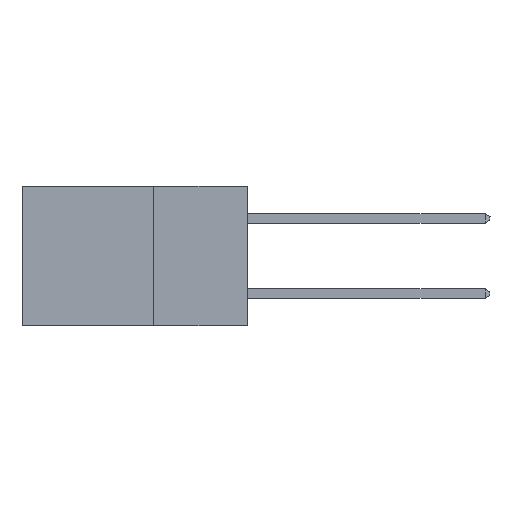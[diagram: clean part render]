
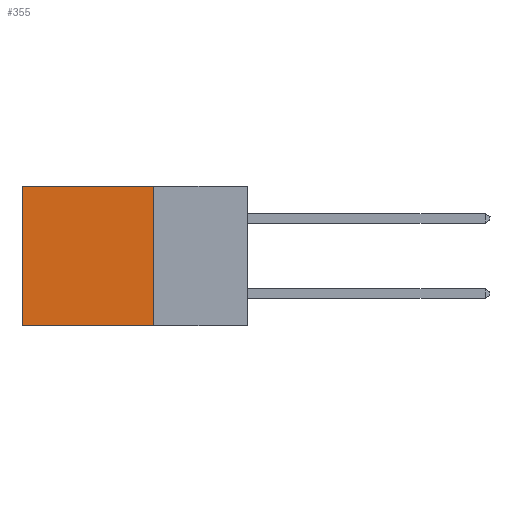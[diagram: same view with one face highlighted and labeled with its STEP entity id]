
A CAD part, left-side view. The second image highlights one B-rep face of the part: STEP entity #355.
In plain terms, the highlighted planar face has unit normal (-1, 0, 0).
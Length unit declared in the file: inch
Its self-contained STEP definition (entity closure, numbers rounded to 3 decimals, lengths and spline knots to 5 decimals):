
#151 = EDGE_CURVE ( 'NONE', #7966, #12110, #7622, .T. ) ;
#355 = ADVANCED_FACE ( 'NONE', ( #9248 ), #10595, .F. ) ;
#1517 = DIRECTION ( 'NONE',  ( 0., 1., 0. ) ) ;
#2015 = EDGE_LOOP ( 'NONE', ( #2437, #8080, #8118, #6639 ) ) ;
#2432 = VERTEX_POINT ( 'NONE', #17488 ) ;
#2437 = ORIENTED_EDGE ( 'NONE', *, *, #8890, .T. ) ;
#2986 = CARTESIAN_POINT ( 'NONE',  ( 0.2615, 0.25, -0.37 ) ) ;
#3216 = VECTOR ( 'NONE', #7838, 39.37008 ) ;
#3565 = DIRECTION ( 'NONE',  ( 1., 0., 0. ) ) ;
#3837 = CARTESIAN_POINT ( 'NONE',  ( 0.2615, 0.25, -0.37 ) ) ;
#6639 = ORIENTED_EDGE ( 'NONE', *, *, #10922, .T. ) ;
#6640 = EDGE_CURVE ( 'NONE', #12110, #2432, #9597, .T. ) ;
#7526 = CARTESIAN_POINT ( 'NONE',  ( 0.2615, 0.25, -0.37 ) ) ;
#7622 = LINE ( 'NONE', #10153, #12758 ) ;
#7838 = DIRECTION ( 'NONE',  ( 0., 0., -1. ) ) ;
#7901 = DIRECTION ( 'NONE',  ( 0., 0., -1. ) ) ;
#7966 = VERTEX_POINT ( 'NONE', #17689 ) ;
#8080 = ORIENTED_EDGE ( 'NONE', *, *, #6640, .F. ) ;
#8118 = ORIENTED_EDGE ( 'NONE', *, *, #151, .F. ) ;
#8156 = DIRECTION ( 'NONE',  ( 0., 1., 0. ) ) ;
#8334 = CARTESIAN_POINT ( 'NONE',  ( 0.2615, 0.6, -0.37 ) ) ;
#8890 = EDGE_CURVE ( 'NONE', #13367, #2432, #16717, .T. ) ;
#9248 = FACE_OUTER_BOUND ( 'NONE', #2015, .T. ) ;
#9597 = LINE ( 'NONE', #2986, #14702 ) ;
#10153 = CARTESIAN_POINT ( 'NONE',  ( 0.2615, 0.25, -0.37 ) ) ;
#10329 = DIRECTION ( 'NONE',  ( 0., 0., -1. ) ) ;
#10595 = PLANE ( 'NONE',  #13626 ) ;
#10922 = EDGE_CURVE ( 'NONE', #7966, #13367, #15314, .T. ) ;
#12110 = VERTEX_POINT ( 'NONE', #7526 ) ;
#12464 = CARTESIAN_POINT ( 'NONE',  ( 0.2615, 0.6, 0. ) ) ;
#12758 = VECTOR ( 'NONE', #10329, 39.37008 ) ;
#13367 = VERTEX_POINT ( 'NONE', #12464 ) ;
#13626 = AXIS2_PLACEMENT_3D ( 'NONE', #3837, #3565, #7901 ) ;
#13871 = CARTESIAN_POINT ( 'NONE',  ( 0.2615, 0.25, 0. ) ) ;
#14702 = VECTOR ( 'NONE', #8156, 39.37008 ) ;
#15314 = LINE ( 'NONE', #13871, #17463 ) ;
#16717 = LINE ( 'NONE', #8334, #3216 ) ;
#17463 = VECTOR ( 'NONE', #1517, 39.37008 ) ;
#17488 = CARTESIAN_POINT ( 'NONE',  ( 0.2615, 0.6, -0.37 ) ) ;
#17689 = CARTESIAN_POINT ( 'NONE',  ( 0.2615, 0.25, 0. ) ) ;
